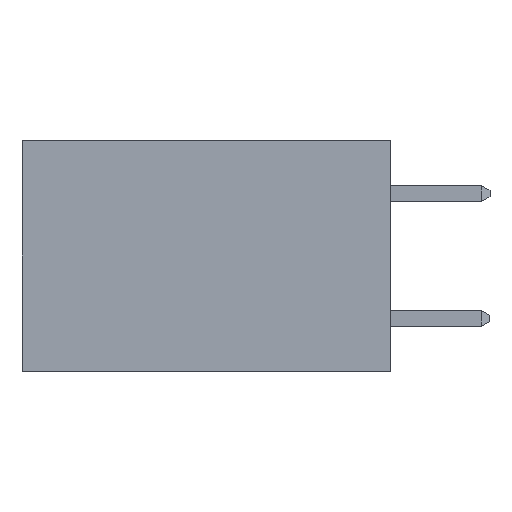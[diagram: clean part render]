
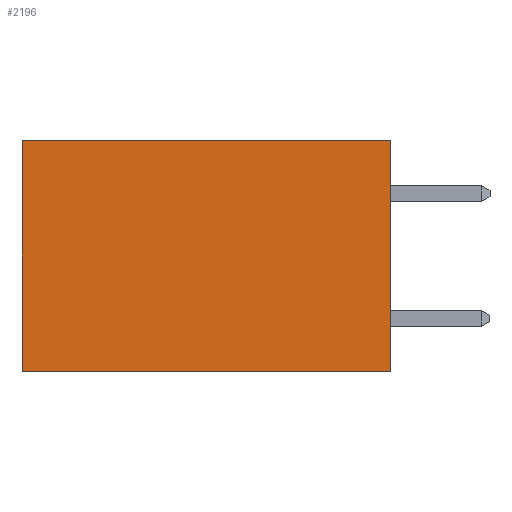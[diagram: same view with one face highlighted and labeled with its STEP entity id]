
A CAD part, left-side view. The second image highlights one B-rep face of the part: STEP entity #2196.
In plain terms, the highlighted planar face has unit normal (-1, 0, 0).
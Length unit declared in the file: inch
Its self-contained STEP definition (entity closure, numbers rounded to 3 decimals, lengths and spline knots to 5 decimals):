
#18 = VECTOR ( 'NONE', #4425, 39.37008 ) ;
#42 = CARTESIAN_POINT ( 'NONE',  ( 0.277, 0., 0. ) ) ;
#613 = DIRECTION ( 'NONE',  ( 0., 0., -1. ) ) ;
#1343 = VERTEX_POINT ( 'NONE', #8637 ) ;
#1452 = DIRECTION ( 'NONE',  ( 1., 0., 0. ) ) ;
#1463 = CARTESIAN_POINT ( 'NONE',  ( 0.277, 0.59, -0.37 ) ) ;
#1473 = EDGE_CURVE ( 'NONE', #1343, #1645, #7910, .T. ) ;
#1645 = VERTEX_POINT ( 'NONE', #7353 ) ;
#1902 = CARTESIAN_POINT ( 'NONE',  ( 0.277, 0., -0.37 ) ) ;
#2145 = PLANE ( 'NONE',  #6270 ) ;
#2196 = ADVANCED_FACE ( 'NONE', ( #7793 ), #2145, .F. ) ;
#2246 = EDGE_CURVE ( 'NONE', #8022, #4921, #5720, .T. ) ;
#2249 = DIRECTION ( 'NONE',  ( 0., 0., -1. ) ) ;
#2375 = VECTOR ( 'NONE', #7649, 39.37008 ) ;
#3378 = EDGE_CURVE ( 'NONE', #4921, #1645, #6704, .T. ) ;
#3971 = EDGE_CURVE ( 'NONE', #8022, #1343, #4498, .T. ) ;
#4160 = VECTOR ( 'NONE', #613, 39.37008 ) ;
#4425 = DIRECTION ( 'NONE',  ( 0., 1., 0. ) ) ;
#4498 = LINE ( 'NONE', #7585, #2375 ) ;
#4921 = VERTEX_POINT ( 'NONE', #7945 ) ;
#5720 = LINE ( 'NONE', #42, #18 ) ;
#6071 = CARTESIAN_POINT ( 'NONE',  ( 0.277, 0., 0. ) ) ;
#6077 = VECTOR ( 'NONE', #8310, 39.37008 ) ;
#6270 = AXIS2_PLACEMENT_3D ( 'NONE', #1902, #1452, #2249 ) ;
#6704 = LINE ( 'NONE', #1463, #4160 ) ;
#6788 = ORIENTED_EDGE ( 'NONE', *, *, #3378, .T. ) ;
#7103 = CARTESIAN_POINT ( 'NONE',  ( 0.277, 0., -0.37 ) ) ;
#7190 = ORIENTED_EDGE ( 'NONE', *, *, #1473, .F. ) ;
#7246 = ORIENTED_EDGE ( 'NONE', *, *, #3971, .F. ) ;
#7353 = CARTESIAN_POINT ( 'NONE',  ( 0.277, 0.59, -0.37 ) ) ;
#7585 = CARTESIAN_POINT ( 'NONE',  ( 0.277, 0., -0.37 ) ) ;
#7649 = DIRECTION ( 'NONE',  ( 0., 0., -1. ) ) ;
#7793 = FACE_OUTER_BOUND ( 'NONE', #8751, .T. ) ;
#7910 = LINE ( 'NONE', #7103, #6077 ) ;
#7945 = CARTESIAN_POINT ( 'NONE',  ( 0.277, 0.59, 0. ) ) ;
#8022 = VERTEX_POINT ( 'NONE', #6071 ) ;
#8310 = DIRECTION ( 'NONE',  ( 0., 1., 0. ) ) ;
#8637 = CARTESIAN_POINT ( 'NONE',  ( 0.277, 0., -0.37 ) ) ;
#8751 = EDGE_LOOP ( 'NONE', ( #6788, #7190, #7246, #8997 ) ) ;
#8997 = ORIENTED_EDGE ( 'NONE', *, *, #2246, .T. ) ;
